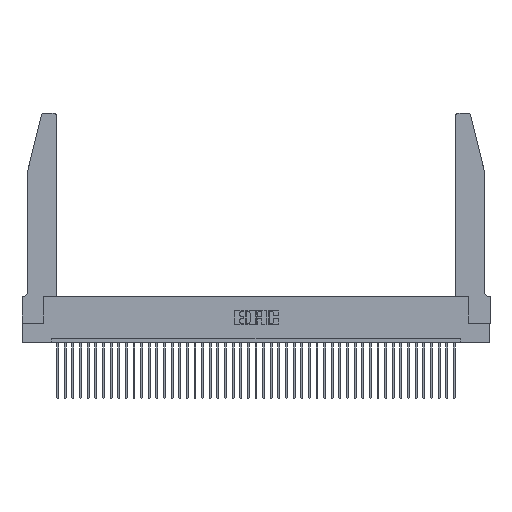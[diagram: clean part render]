
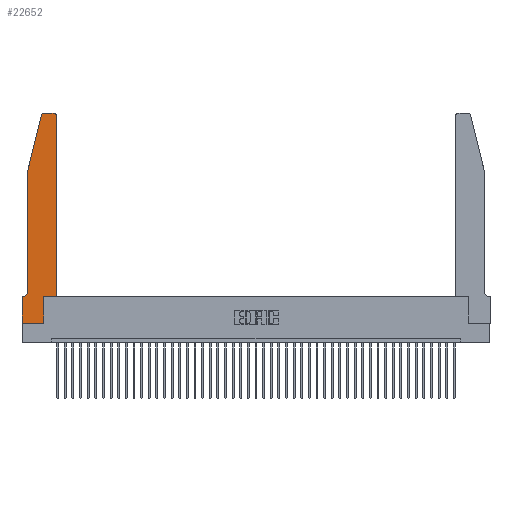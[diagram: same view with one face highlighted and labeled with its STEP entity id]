
A CAD part, top view. The second image highlights one B-rep face of the part: STEP entity #22652.
In plain terms, the highlighted planar face has unit normal (0, 0, 1).
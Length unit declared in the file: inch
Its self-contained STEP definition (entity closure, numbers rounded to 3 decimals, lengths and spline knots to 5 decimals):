
#847 = DIRECTION ( 'NONE',  ( 1., 0., 0. ) ) ;
#1458 = CARTESIAN_POINT ( 'NONE',  ( 0.2865, 0., 0.37 ) ) ;
#1524 = EDGE_CURVE ( 'NONE', #8160, #32919, #27115, .T. ) ;
#3732 = CARTESIAN_POINT ( 'NONE',  ( 0.2605, 2.75, 0.37 ) ) ;
#3738 = LINE ( 'NONE', #26916, #23517 ) ;
#3809 = ORIENTED_EDGE ( 'NONE', *, *, #32215, .T. ) ;
#4098 = DIRECTION ( 'NONE',  ( 0., -1., 0. ) ) ;
#4105 = EDGE_CURVE ( 'NONE', #38444, #17312, #23157, .T. ) ;
#4340 = DIRECTION ( 'NONE',  ( -1., 0., 0. ) ) ;
#4403 = VERTEX_POINT ( 'NONE', #14022 ) ;
#4558 = DIRECTION ( 'NONE',  ( 1., 0., 0. ) ) ;
#4770 = CARTESIAN_POINT ( 'NONE',  ( 0., 0., 0.37 ) ) ;
#4876 = ORIENTED_EDGE ( 'NONE', *, *, #21427, .T. ) ;
#5907 = EDGE_CURVE ( 'NONE', #42866, #16609, #26701, .T. ) ;
#6371 = DIRECTION ( 'NONE',  ( -1., 0., 0. ) ) ;
#6418 = LINE ( 'NONE', #12727, #27251 ) ;
#6602 = CARTESIAN_POINT ( 'NONE',  ( 0.284, 2.75, 0.37 ) ) ;
#6972 = DIRECTION ( 'NONE',  ( 0., 1., 0. ) ) ;
#7245 = VECTOR ( 'NONE', #12645, 39.37008 ) ;
#7989 = ORIENTED_EDGE ( 'NONE', *, *, #34651, .T. ) ;
#8160 = VERTEX_POINT ( 'NONE', #28171 ) ;
#8295 = LINE ( 'NONE', #3732, #20774 ) ;
#8886 = DIRECTION ( 'NONE',  ( 1., 0., 0. ) ) ;
#9016 = ORIENTED_EDGE ( 'NONE', *, *, #22194, .T. ) ;
#11395 = DIRECTION ( 'NONE',  ( 0., -1., 0. ) ) ;
#12128 = EDGE_CURVE ( 'NONE', #32919, #12820, #36723, .T. ) ;
#12645 = DIRECTION ( 'NONE',  ( 0., 1., 0. ) ) ;
#12679 = ORIENTED_EDGE ( 'NONE', *, *, #12128, .T. ) ;
#12727 = CARTESIAN_POINT ( 'NONE',  ( 0.0755, 2., 0.37 ) ) ;
#12820 = VERTEX_POINT ( 'NONE', #4770 ) ;
#13696 = CARTESIAN_POINT ( 'NONE',  ( 0.2865, 0.35, 0.37 ) ) ;
#14022 = CARTESIAN_POINT ( 'NONE',  ( 0.25487, 2.72718, 0.37 ) ) ;
#15316 = CARTESIAN_POINT ( 'NONE',  ( 0.284, 2.72, 0.37 ) ) ;
#16443 = CARTESIAN_POINT ( 'NONE',  ( 0.0755, 0.42, 0.37 ) ) ;
#16523 = PLANE ( 'NONE',  #24044 ) ;
#16609 = VERTEX_POINT ( 'NONE', #21253 ) ;
#17098 = CARTESIAN_POINT ( 'NONE',  ( 0.4505, 0.35, 0.37 ) ) ;
#17312 = VERTEX_POINT ( 'NONE', #16443 ) ;
#18240 = VECTOR ( 'NONE', #30907, 39.37008 ) ;
#18470 = DIRECTION ( 'NONE',  ( 1., 0., 0. ) ) ;
#18961 = DIRECTION ( 'NONE',  ( -0.239, -0.971, 0. ) ) ;
#19490 = VERTEX_POINT ( 'NONE', #1458 ) ;
#19576 = CARTESIAN_POINT ( 'NONE',  ( 0., 0.35, 0.37 ) ) ;
#20575 = CARTESIAN_POINT ( 'NONE',  ( 0.0755, 0.35, 0.37 ) ) ;
#20774 = VECTOR ( 'NONE', #6371, 39.37008 ) ;
#20785 = CARTESIAN_POINT ( 'NONE',  ( 0.4505, 2.72, 0.37 ) ) ;
#21253 = CARTESIAN_POINT ( 'NONE',  ( 0.4205, 2.75, 0.37 ) ) ;
#21427 = EDGE_CURVE ( 'NONE', #17312, #8160, #28823, .T. ) ;
#21522 = EDGE_LOOP ( 'NONE', ( #24303, #9016, #26907, #42544, #4876, #26188, #12679, #7989, #39611, #3809, #25014, #31266 ) ) ;
#21577 = CARTESIAN_POINT ( 'NONE',  ( 0., 0., 0.37 ) ) ;
#21839 = LINE ( 'NONE', #32852, #7245 ) ;
#22194 = EDGE_CURVE ( 'NONE', #38038, #4403, #40723, .T. ) ;
#22652 = ADVANCED_FACE ( 'NONE', ( #22989 ), #16523, .T. ) ;
#22989 = FACE_OUTER_BOUND ( 'NONE', #21522, .T. ) ;
#23014 = VECTOR ( 'NONE', #847, 39.37008 ) ;
#23157 = LINE ( 'NONE', #40486, #38257 ) ;
#23226 = DIRECTION ( 'NONE',  ( 1., 0., 0. ) ) ;
#23517 = VECTOR ( 'NONE', #6972, 39.37008 ) ;
#24044 = AXIS2_PLACEMENT_3D ( 'NONE', #19576, #39837, #23226 ) ;
#24303 = ORIENTED_EDGE ( 'NONE', *, *, #39219, .T. ) ;
#25014 = ORIENTED_EDGE ( 'NONE', *, *, #39178, .T. ) ;
#26188 = ORIENTED_EDGE ( 'NONE', *, *, #1524, .T. ) ;
#26423 = VECTOR ( 'NONE', #4558, 39.37008 ) ;
#26701 = CIRCLE ( 'NONE', #41969, 0.03 ) ;
#26907 = ORIENTED_EDGE ( 'NONE', *, *, #27394, .T. ) ;
#26916 = CARTESIAN_POINT ( 'NONE',  ( 0.2865, 0.35, 0.37 ) ) ;
#27115 = LINE ( 'NONE', #20575, #18240 ) ;
#27251 = VECTOR ( 'NONE', #18961, 39.37008 ) ;
#27394 = EDGE_CURVE ( 'NONE', #4403, #38444, #6418, .T. ) ;
#28171 = CARTESIAN_POINT ( 'NONE',  ( 0.0055, 0.35, 0.37 ) ) ;
#28823 = CIRCLE ( 'NONE', #32560, 0.07 ) ;
#28978 = DIRECTION ( 'NONE',  ( 0., 0., 1. ) ) ;
#30409 = DIRECTION ( 'NONE',  ( 0., 0., -1. ) ) ;
#30821 = CARTESIAN_POINT ( 'NONE',  ( 0.0055, 0.42, 0.37 ) ) ;
#30907 = DIRECTION ( 'NONE',  ( -1., 0., 0. ) ) ;
#31266 = ORIENTED_EDGE ( 'NONE', *, *, #5907, .T. ) ;
#32215 = EDGE_CURVE ( 'NONE', #38168, #35272, #42837, .T. ) ;
#32560 = AXIS2_PLACEMENT_3D ( 'NONE', #30821, #30409, #4340 ) ;
#32573 = VECTOR ( 'NONE', #11395, 39.37008 ) ;
#32852 = CARTESIAN_POINT ( 'NONE',  ( 0.4505, 0.35, 0.37 ) ) ;
#32919 = VERTEX_POINT ( 'NONE', #33307 ) ;
#33212 = AXIS2_PLACEMENT_3D ( 'NONE', #15316, #35233, #8886 ) ;
#33307 = CARTESIAN_POINT ( 'NONE',  ( 0., 0.35, 0.37 ) ) ;
#34202 = EDGE_CURVE ( 'NONE', #19490, #38168, #3738, .T. ) ;
#34346 = CARTESIAN_POINT ( 'NONE',  ( 0., 0., 0.37 ) ) ;
#34651 = EDGE_CURVE ( 'NONE', #12820, #19490, #35231, .T. ) ;
#35231 = LINE ( 'NONE', #21577, #26423 ) ;
#35233 = DIRECTION ( 'NONE',  ( 0., 0., 1. ) ) ;
#35272 = VERTEX_POINT ( 'NONE', #17098 ) ;
#35521 = CARTESIAN_POINT ( 'NONE',  ( 0.0755, 2., 0.37 ) ) ;
#35642 = CARTESIAN_POINT ( 'NONE',  ( 0.4205, 2.72, 0.37 ) ) ;
#36723 = LINE ( 'NONE', #34346, #32573 ) ;
#38026 = CARTESIAN_POINT ( 'NONE',  ( 0.4505, 0.35, 0.37 ) ) ;
#38038 = VERTEX_POINT ( 'NONE', #6602 ) ;
#38168 = VERTEX_POINT ( 'NONE', #13696 ) ;
#38257 = VECTOR ( 'NONE', #4098, 39.37008 ) ;
#38444 = VERTEX_POINT ( 'NONE', #35521 ) ;
#39178 = EDGE_CURVE ( 'NONE', #35272, #42866, #21839, .T. ) ;
#39219 = EDGE_CURVE ( 'NONE', #16609, #38038, #8295, .T. ) ;
#39611 = ORIENTED_EDGE ( 'NONE', *, *, #34202, .T. ) ;
#39837 = DIRECTION ( 'NONE',  ( 0., 0., 1. ) ) ;
#40486 = CARTESIAN_POINT ( 'NONE',  ( 0.0755, 2., 0.37 ) ) ;
#40723 = CIRCLE ( 'NONE', #33212, 0.03 ) ;
#41969 = AXIS2_PLACEMENT_3D ( 'NONE', #35642, #28978, #18470 ) ;
#42544 = ORIENTED_EDGE ( 'NONE', *, *, #4105, .T. ) ;
#42837 = LINE ( 'NONE', #38026, #23014 ) ;
#42866 = VERTEX_POINT ( 'NONE', #20785 ) ;
